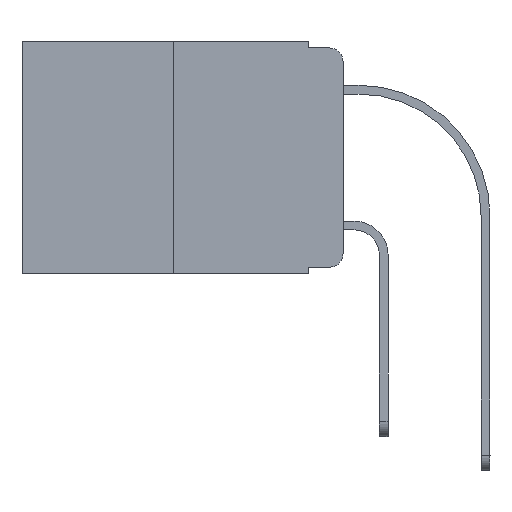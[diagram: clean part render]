
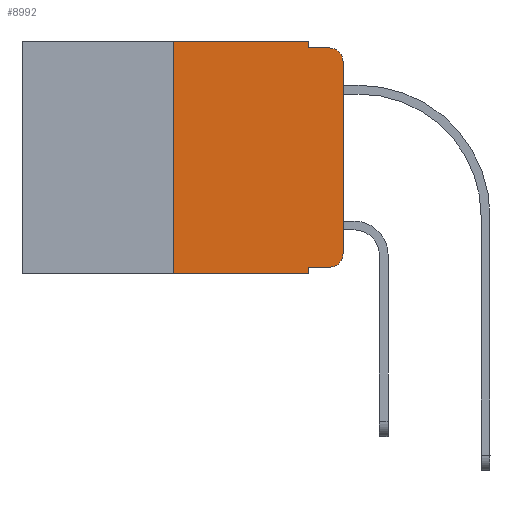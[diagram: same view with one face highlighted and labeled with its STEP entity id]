
A CAD part, left-side view. The second image highlights one B-rep face of the part: STEP entity #8992.
In plain terms, the highlighted planar face has unit normal (-1, 0, 0).
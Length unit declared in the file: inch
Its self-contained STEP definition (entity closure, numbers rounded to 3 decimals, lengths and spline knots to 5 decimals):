
#128 = AXIS2_PLACEMENT_3D ( 'NONE', #9248, #15326, #11450 ) ;
#172 = CARTESIAN_POINT ( 'NONE',  ( 0., 0.051, 0. ) ) ;
#228 = EDGE_CURVE ( 'NONE', #18569, #4723, #12994, .T. ) ;
#235 = EDGE_CURVE ( 'NONE', #3475, #15601, #6909, .T. ) ;
#921 = CARTESIAN_POINT ( 'NONE',  ( 0., 0.25, 0. ) ) ;
#934 = CARTESIAN_POINT ( 'NONE',  ( 0., 0.051, -0.01 ) ) ;
#1123 = CARTESIAN_POINT ( 'NONE',  ( 0., 0., 0. ) ) ;
#1236 = AXIS2_PLACEMENT_3D ( 'NONE', #18353, #15280, #1840 ) ;
#1785 = ORIENTED_EDGE ( 'NONE', *, *, #235, .F. ) ;
#1802 = CARTESIAN_POINT ( 'NONE',  ( 0., 0.051, -0.01 ) ) ;
#1816 = EDGE_CURVE ( 'NONE', #3207, #5861, #11176, .T. ) ;
#1840 = DIRECTION ( 'NONE',  ( 0., 0., -1. ) ) ;
#1865 = LINE ( 'NONE', #10834, #11241 ) ;
#2995 = CIRCLE ( 'NONE', #128, 0.02 ) ;
#3207 = VERTEX_POINT ( 'NONE', #921 ) ;
#3475 = VERTEX_POINT ( 'NONE', #1802 ) ;
#3596 = CARTESIAN_POINT ( 'NONE',  ( 0., 0., -0.313 ) ) ;
#3656 = CARTESIAN_POINT ( 'NONE',  ( 0., 0., -0.03 ) ) ;
#3812 = CARTESIAN_POINT ( 'NONE',  ( 0., 0.02, -0.313 ) ) ;
#3997 = CARTESIAN_POINT ( 'NONE',  ( 0., 0.25, -0.343 ) ) ;
#4502 = VERTEX_POINT ( 'NONE', #3656 ) ;
#4583 = VECTOR ( 'NONE', #17548, 39.37008 ) ;
#4723 = VERTEX_POINT ( 'NONE', #13970 ) ;
#4743 = ORIENTED_EDGE ( 'NONE', *, *, #13161, .T. ) ;
#5014 = CARTESIAN_POINT ( 'NONE',  ( 0., 0.25, 0. ) ) ;
#5782 = DIRECTION ( 'NONE',  ( 0., -1., 0. ) ) ;
#5861 = VERTEX_POINT ( 'NONE', #172 ) ;
#5899 = ORIENTED_EDGE ( 'NONE', *, *, #7190, .F. ) ;
#6309 = CIRCLE ( 'NONE', #17417, 0.02 ) ;
#6909 = LINE ( 'NONE', #934, #4583 ) ;
#7089 = DIRECTION ( 'NONE',  ( 0., 0., -1. ) ) ;
#7132 = VECTOR ( 'NONE', #13199, 39.37008 ) ;
#7190 = EDGE_CURVE ( 'NONE', #18569, #8658, #1865, .T. ) ;
#7695 = VECTOR ( 'NONE', #5782, 39.37008 ) ;
#8166 = ORIENTED_EDGE ( 'NONE', *, *, #8792, .F. ) ;
#8658 = VERTEX_POINT ( 'NONE', #9455 ) ;
#8792 = EDGE_CURVE ( 'NONE', #5861, #3475, #11924, .T. ) ;
#8992 = ADVANCED_FACE ( 'NONE', ( #18548 ), #13691, .F. ) ;
#9248 = CARTESIAN_POINT ( 'NONE',  ( 0., 0.02, -0.03 ) ) ;
#9455 = CARTESIAN_POINT ( 'NONE',  ( 0., 0.051, -0.343 ) ) ;
#9872 = DIRECTION ( 'NONE',  ( -1., 0., 0. ) ) ;
#10211 = ORIENTED_EDGE ( 'NONE', *, *, #17966, .F. ) ;
#10268 = VECTOR ( 'NONE', #15862, 39.37008 ) ;
#10405 = ORIENTED_EDGE ( 'NONE', *, *, #1816, .F. ) ;
#10452 = CARTESIAN_POINT ( 'NONE',  ( 0., 0.473, -0.343 ) ) ;
#10834 = CARTESIAN_POINT ( 'NONE',  ( 0., 0.051, 0. ) ) ;
#11176 = LINE ( 'NONE', #18925, #10268 ) ;
#11241 = VECTOR ( 'NONE', #13822, 39.37008 ) ;
#11450 = DIRECTION ( 'NONE',  ( 0., 0., -1. ) ) ;
#11783 = DIRECTION ( 'NONE',  ( 0., 0., 1. ) ) ;
#11812 = EDGE_CURVE ( 'NONE', #4723, #13899, #6309, .T. ) ;
#11924 = LINE ( 'NONE', #19648, #17425 ) ;
#12136 = CARTESIAN_POINT ( 'NONE',  ( 0., 0.051, -0.333 ) ) ;
#12214 = ORIENTED_EDGE ( 'NONE', *, *, #228, .T. ) ;
#12260 = EDGE_LOOP ( 'NONE', ( #4743, #16690, #1785, #8166, #10405, #10211, #17383, #5899, #12214, #13611 ) ) ;
#12672 = DIRECTION ( 'NONE',  ( 0., 0., 1. ) ) ;
#12994 = LINE ( 'NONE', #18938, #7132 ) ;
#13161 = EDGE_CURVE ( 'NONE', #13899, #4502, #18922, .T. ) ;
#13199 = DIRECTION ( 'NONE',  ( 0., -1., 0. ) ) ;
#13611 = ORIENTED_EDGE ( 'NONE', *, *, #11812, .T. ) ;
#13691 = PLANE ( 'NONE',  #1236 ) ;
#13822 = DIRECTION ( 'NONE',  ( 0., 0., -1. ) ) ;
#13899 = VERTEX_POINT ( 'NONE', #3596 ) ;
#13970 = CARTESIAN_POINT ( 'NONE',  ( 0., 0.02, -0.333 ) ) ;
#14171 = LINE ( 'NONE', #5014, #19477 ) ;
#14705 = DIRECTION ( 'NONE',  ( 0., 0., -1. ) ) ;
#14938 = VECTOR ( 'NONE', #11783, 39.37008 ) ;
#15280 = DIRECTION ( 'NONE',  ( 1., 0., 0. ) ) ;
#15326 = DIRECTION ( 'NONE',  ( -1., 0., 0. ) ) ;
#15601 = VERTEX_POINT ( 'NONE', #18106 ) ;
#15800 = EDGE_CURVE ( 'NONE', #4502, #15601, #2995, .T. ) ;
#15862 = DIRECTION ( 'NONE',  ( 0., -1., 0. ) ) ;
#16690 = ORIENTED_EDGE ( 'NONE', *, *, #15800, .T. ) ;
#17267 = VERTEX_POINT ( 'NONE', #3997 ) ;
#17383 = ORIENTED_EDGE ( 'NONE', *, *, #18636, .T. ) ;
#17417 = AXIS2_PLACEMENT_3D ( 'NONE', #3812, #9872, #7089 ) ;
#17425 = VECTOR ( 'NONE', #14705, 39.37008 ) ;
#17548 = DIRECTION ( 'NONE',  ( 0., -1., 0. ) ) ;
#17966 = EDGE_CURVE ( 'NONE', #17267, #3207, #14171, .T. ) ;
#18000 = LINE ( 'NONE', #10452, #7695 ) ;
#18106 = CARTESIAN_POINT ( 'NONE',  ( 0., 0.02, -0.01 ) ) ;
#18353 = CARTESIAN_POINT ( 'NONE',  ( 0., 0.473, 0. ) ) ;
#18548 = FACE_OUTER_BOUND ( 'NONE', #12260, .T. ) ;
#18569 = VERTEX_POINT ( 'NONE', #12136 ) ;
#18636 = EDGE_CURVE ( 'NONE', #17267, #8658, #18000, .T. ) ;
#18922 = LINE ( 'NONE', #1123, #14938 ) ;
#18925 = CARTESIAN_POINT ( 'NONE',  ( 0., 0.473, 0. ) ) ;
#18938 = CARTESIAN_POINT ( 'NONE',  ( 0., 0.051, -0.333 ) ) ;
#19477 = VECTOR ( 'NONE', #12672, 39.37008 ) ;
#19648 = CARTESIAN_POINT ( 'NONE',  ( 0., 0.051, 0. ) ) ;
